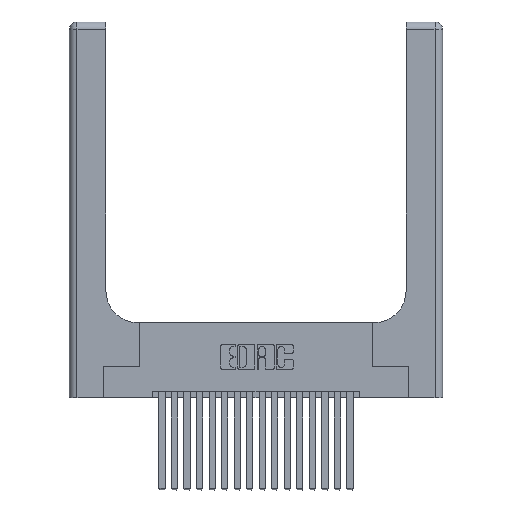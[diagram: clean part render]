
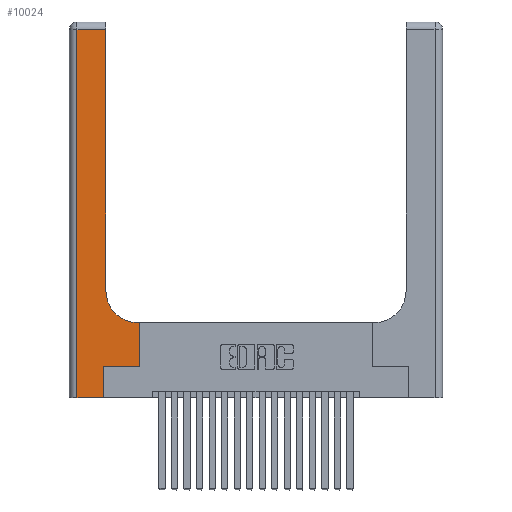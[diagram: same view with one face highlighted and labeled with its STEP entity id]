
A CAD part, top view. The second image highlights one B-rep face of the part: STEP entity #10024.
In plain terms, the highlighted planar face has unit normal (0, 0, 1).
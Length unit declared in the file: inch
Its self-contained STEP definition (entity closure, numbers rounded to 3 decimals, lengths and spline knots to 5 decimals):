
#475 = ORIENTED_EDGE ( 'NONE', *, *, #4955, .T. ) ;
#916 = EDGE_CURVE ( 'NONE', #8992, #20835, #2248, .T. ) ;
#979 = CARTESIAN_POINT ( 'NONE',  ( 0.2915, 3., 0.37 ) ) ;
#1033 = VECTOR ( 'NONE', #11824, 39.37008 ) ;
#1094 = CARTESIAN_POINT ( 'NONE',  ( 0.06, 2.94, 0.37 ) ) ;
#2248 = LINE ( 'NONE', #11499, #15146 ) ;
#2412 = VECTOR ( 'NONE', #4225, 39.37008 ) ;
#2683 = VECTOR ( 'NONE', #16380, 39.37008 ) ;
#2749 = PLANE ( 'NONE',  #7294 ) ;
#3104 = ORIENTED_EDGE ( 'NONE', *, *, #11761, .T. ) ;
#3137 = VECTOR ( 'NONE', #4355, 39.37008 ) ;
#3451 = FACE_OUTER_BOUND ( 'NONE', #10131, .T. ) ;
#4109 = CARTESIAN_POINT ( 'NONE',  ( 0.06, 0., 0.37 ) ) ;
#4115 = CARTESIAN_POINT ( 'NONE',  ( 0.269, 0., 0.37 ) ) ;
#4225 = DIRECTION ( 'NONE',  ( 0., 1., 0. ) ) ;
#4355 = DIRECTION ( 'NONE',  ( 0., 1., 0. ) ) ;
#4922 = VERTEX_POINT ( 'NONE', #14085 ) ;
#4955 = EDGE_CURVE ( 'NONE', #15422, #19468, #16250, .T. ) ;
#5384 = LINE ( 'NONE', #8573, #1033 ) ;
#5785 = EDGE_CURVE ( 'NONE', #19663, #9885, #5384, .T. ) ;
#5876 = VECTOR ( 'NONE', #9099, 39.37008 ) ;
#6039 = DIRECTION ( 'NONE',  ( 0., 0., -1. ) ) ;
#6346 = AXIS2_PLACEMENT_3D ( 'NONE', #16679, #7026, #18339 ) ;
#6367 = LINE ( 'NONE', #979, #5876 ) ;
#6919 = EDGE_CURVE ( 'NONE', #19267, #4922, #6367, .T. ) ;
#7026 = DIRECTION ( 'NONE',  ( 0., 0., -1. ) ) ;
#7294 = AXIS2_PLACEMENT_3D ( 'NONE', #9156, #6039, #17322 ) ;
#7650 = ORIENTED_EDGE ( 'NONE', *, *, #5785, .T. ) ;
#7750 = CIRCLE ( 'NONE', #6346, 0.25 ) ;
#7984 = LINE ( 'NONE', #20528, #3137 ) ;
#8203 = VECTOR ( 'NONE', #20649, 39.37008 ) ;
#8295 = LINE ( 'NONE', #13178, #20717 ) ;
#8470 = ORIENTED_EDGE ( 'NONE', *, *, #12413, .T. ) ;
#8573 = CARTESIAN_POINT ( 'NONE',  ( 0.06, 3., 0.37 ) ) ;
#8992 = VERTEX_POINT ( 'NONE', #11625 ) ;
#9063 = CARTESIAN_POINT ( 'NONE',  ( 0.269, 0., 0.37 ) ) ;
#9099 = DIRECTION ( 'NONE',  ( 0., 1., 0. ) ) ;
#9156 = CARTESIAN_POINT ( 'NONE',  ( 0., 3., 0.37 ) ) ;
#9885 = VERTEX_POINT ( 'NONE', #4109 ) ;
#9992 = CARTESIAN_POINT ( 'NONE',  ( 0., 0., 0.37 ) ) ;
#10024 = ADVANCED_FACE ( 'NONE', ( #3451 ), #2749, .F. ) ;
#10131 = EDGE_LOOP ( 'NONE', ( #13165, #12884, #7650, #16925, #13946, #475, #8470, #13759, #3104 ) ) ;
#10280 = CARTESIAN_POINT ( 'NONE',  ( 0.5585, 0.25, 0.37 ) ) ;
#10301 = EDGE_CURVE ( 'NONE', #9885, #18879, #15584, .T. ) ;
#10550 = EDGE_CURVE ( 'NONE', #18879, #15422, #11067, .T. ) ;
#11067 = LINE ( 'NONE', #9063, #2412 ) ;
#11409 = CARTESIAN_POINT ( 'NONE',  ( 0.2915, 0.85, 0.37 ) ) ;
#11499 = CARTESIAN_POINT ( 'NONE',  ( 0.2915, 0.6, 0.37 ) ) ;
#11625 = CARTESIAN_POINT ( 'NONE',  ( 0.5585, 0.6, 0.37 ) ) ;
#11761 = EDGE_CURVE ( 'NONE', #20835, #19267, #7750, .T. ) ;
#11770 = DIRECTION ( 'NONE',  ( -1., 0., 0. ) ) ;
#11824 = DIRECTION ( 'NONE',  ( 0., -1., 0. ) ) ;
#12413 = EDGE_CURVE ( 'NONE', #19468, #8992, #7984, .T. ) ;
#12884 = ORIENTED_EDGE ( 'NONE', *, *, #18639, .T. ) ;
#13165 = ORIENTED_EDGE ( 'NONE', *, *, #6919, .T. ) ;
#13178 = CARTESIAN_POINT ( 'NONE',  ( 0., 2.94, 0.37 ) ) ;
#13340 = CARTESIAN_POINT ( 'NONE',  ( 0.269, 0.25, 0.37 ) ) ;
#13759 = ORIENTED_EDGE ( 'NONE', *, *, #916, .T. ) ;
#13946 = ORIENTED_EDGE ( 'NONE', *, *, #10550, .T. ) ;
#14085 = CARTESIAN_POINT ( 'NONE',  ( 0.2915, 2.94, 0.37 ) ) ;
#14153 = CARTESIAN_POINT ( 'NONE',  ( 0.269, 0.25, 0.37 ) ) ;
#14763 = DIRECTION ( 'NONE',  ( -1., 0., 0. ) ) ;
#15146 = VECTOR ( 'NONE', #11770, 39.37008 ) ;
#15422 = VERTEX_POINT ( 'NONE', #13340 ) ;
#15584 = LINE ( 'NONE', #9992, #2683 ) ;
#16250 = LINE ( 'NONE', #14153, #8203 ) ;
#16380 = DIRECTION ( 'NONE',  ( 1., 0., 0. ) ) ;
#16679 = CARTESIAN_POINT ( 'NONE',  ( 0.5415, 0.85, 0.37 ) ) ;
#16925 = ORIENTED_EDGE ( 'NONE', *, *, #10301, .T. ) ;
#17322 = DIRECTION ( 'NONE',  ( -1., 0., 0. ) ) ;
#18339 = DIRECTION ( 'NONE',  ( 1., 0., 0. ) ) ;
#18639 = EDGE_CURVE ( 'NONE', #4922, #19663, #8295, .T. ) ;
#18879 = VERTEX_POINT ( 'NONE', #4115 ) ;
#19267 = VERTEX_POINT ( 'NONE', #11409 ) ;
#19468 = VERTEX_POINT ( 'NONE', #10280 ) ;
#19535 = CARTESIAN_POINT ( 'NONE',  ( 0.5415, 0.6, 0.37 ) ) ;
#19663 = VERTEX_POINT ( 'NONE', #1094 ) ;
#20528 = CARTESIAN_POINT ( 'NONE',  ( 0.5585, 0.25, 0.37 ) ) ;
#20649 = DIRECTION ( 'NONE',  ( 1., 0., 0. ) ) ;
#20717 = VECTOR ( 'NONE', #14763, 39.37008 ) ;
#20835 = VERTEX_POINT ( 'NONE', #19535 ) ;
